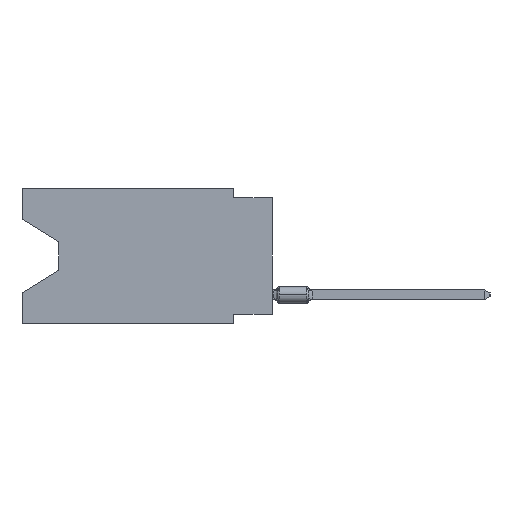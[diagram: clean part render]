
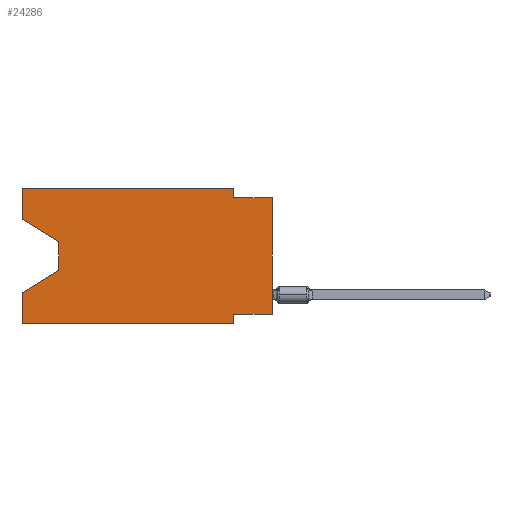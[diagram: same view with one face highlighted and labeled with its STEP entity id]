
A CAD part, left-side view. The second image highlights one B-rep face of the part: STEP entity #24286.
In plain terms, the highlighted planar face has unit normal (-1, 0, 0).
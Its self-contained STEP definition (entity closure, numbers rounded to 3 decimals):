
#262 = VECTOR ( 'NONE', #4071, 1000. ) ;
#324 = ORIENTED_EDGE ( 'NONE', *, *, #18573, .F. ) ;
#328 = CARTESIAN_POINT ( 'NONE',  ( 0., 16.383, -2.038 ) ) ;
#471 = LINE ( 'NONE', #13363, #9251 ) ;
#623 = PLANE ( 'NONE',  #5775 ) ;
#1856 = LINE ( 'NONE', #10464, #262 ) ;
#2342 = EDGE_CURVE ( 'NONE', #5266, #21382, #18797, .T. ) ;
#2840 = CARTESIAN_POINT ( 'NONE',  ( 0., 2.54, 0. ) ) ;
#3054 = LINE ( 'NONE', #19985, #20919 ) ;
#3543 = DIRECTION ( 'NONE',  ( 0., 0., -1. ) ) ;
#4071 = DIRECTION ( 'NONE',  ( 0., 0., 1. ) ) ;
#4153 = CARTESIAN_POINT ( 'NONE',  ( 0., 13.97, -5.385 ) ) ;
#4239 = DIRECTION ( 'NONE',  ( 0., 1., 0. ) ) ;
#4320 = CARTESIAN_POINT ( 'NONE',  ( 0., 0., -0.635 ) ) ;
#4401 = VERTEX_POINT ( 'NONE', #4153 ) ;
#4506 = CARTESIAN_POINT ( 'NONE',  ( 0., 2.54, -8.255 ) ) ;
#4637 = FACE_OUTER_BOUND ( 'NONE', #16215, .T. ) ;
#5173 = EDGE_CURVE ( 'NONE', #19352, #20812, #471, .T. ) ;
#5266 = VERTEX_POINT ( 'NONE', #328 ) ;
#5278 = VECTOR ( 'NONE', #3543, 1000. ) ;
#5775 = AXIS2_PLACEMENT_3D ( 'NONE', #13106, #11027, #21830 ) ;
#6265 = CARTESIAN_POINT ( 'NONE',  ( 0., 16.383, 0. ) ) ;
#6317 = DIRECTION ( 'NONE',  ( 0., -0.855, -0.519 ) ) ;
#6506 = VECTOR ( 'NONE', #14333, 1000. ) ;
#6592 = ORIENTED_EDGE ( 'NONE', *, *, #15731, .T. ) ;
#7139 = VECTOR ( 'NONE', #4239, 1000. ) ;
#7434 = LINE ( 'NONE', #18246, #5278 ) ;
#7458 = EDGE_CURVE ( 'NONE', #15895, #26619, #1856, .T. ) ;
#7667 = CARTESIAN_POINT ( 'NONE',  ( 0., 16.383, 0. ) ) ;
#7800 = LINE ( 'NONE', #11977, #6506 ) ;
#7867 = CARTESIAN_POINT ( 'NONE',  ( 0., 16.383, -8.89 ) ) ;
#8213 = ORIENTED_EDGE ( 'NONE', *, *, #8939, .F. ) ;
#8368 = LINE ( 'NONE', #10178, #14733 ) ;
#8939 = EDGE_CURVE ( 'NONE', #5266, #10581, #8368, .T. ) ;
#8975 = ORIENTED_EDGE ( 'NONE', *, *, #22184, .F. ) ;
#9251 = VECTOR ( 'NONE', #21412, 1000. ) ;
#9270 = VECTOR ( 'NONE', #25116, 1000. ) ;
#9853 = CARTESIAN_POINT ( 'NONE',  ( 0., 2.54, -0.635 ) ) ;
#9855 = CARTESIAN_POINT ( 'NONE',  ( 0., 2.54, -8.89 ) ) ;
#10178 = CARTESIAN_POINT ( 'NONE',  ( 0., 16.383, 0. ) ) ;
#10286 = EDGE_CURVE ( 'NONE', #10581, #26738, #18322, .T. ) ;
#10464 = CARTESIAN_POINT ( 'NONE',  ( 0., 0., 0. ) ) ;
#10512 = EDGE_CURVE ( 'NONE', #19696, #26619, #23321, .T. ) ;
#10581 = VERTEX_POINT ( 'NONE', #7667 ) ;
#10823 = VECTOR ( 'NONE', #12796, 1000. ) ;
#11027 = DIRECTION ( 'NONE',  ( 1., 0., 0. ) ) ;
#11950 = ORIENTED_EDGE ( 'NONE', *, *, #10286, .F. ) ;
#11977 = CARTESIAN_POINT ( 'NONE',  ( 0., 13.97, -5.385 ) ) ;
#12538 = DIRECTION ( 'NONE',  ( 0., 0., 1. ) ) ;
#12659 = LINE ( 'NONE', #6265, #9270 ) ;
#12776 = ORIENTED_EDGE ( 'NONE', *, *, #2342, .T. ) ;
#12796 = DIRECTION ( 'NONE',  ( 0., -1., 0. ) ) ;
#13106 = CARTESIAN_POINT ( 'NONE',  ( 0., 16.383, 0. ) ) ;
#13363 = CARTESIAN_POINT ( 'NONE',  ( 0., 16.383, -8.89 ) ) ;
#13785 = LINE ( 'NONE', #18331, #18627 ) ;
#14333 = DIRECTION ( 'NONE',  ( 0., 0.855, -0.519 ) ) ;
#14733 = VECTOR ( 'NONE', #12538, 1000. ) ;
#15122 = ORIENTED_EDGE ( 'NONE', *, *, #20645, .F. ) ;
#15731 = EDGE_CURVE ( 'NONE', #4401, #20857, #7800, .T. ) ;
#15895 = VERTEX_POINT ( 'NONE', #27357 ) ;
#16215 = EDGE_LOOP ( 'NONE', ( #12776, #17631, #6592, #8975, #17224, #324, #15122, #19209, #16489, #25407, #11950, #8213 ) ) ;
#16489 = ORIENTED_EDGE ( 'NONE', *, *, #10512, .F. ) ;
#17175 = CARTESIAN_POINT ( 'NONE',  ( 0., 13.97, -3.505 ) ) ;
#17224 = ORIENTED_EDGE ( 'NONE', *, *, #5173, .T. ) ;
#17631 = ORIENTED_EDGE ( 'NONE', *, *, #21135, .T. ) ;
#18037 = VECTOR ( 'NONE', #6317, 1000. ) ;
#18246 = CARTESIAN_POINT ( 'NONE',  ( 0., 2.54, -8.89 ) ) ;
#18322 = LINE ( 'NONE', #22482, #24961 ) ;
#18331 = CARTESIAN_POINT ( 'NONE',  ( 0., 2.54, 0. ) ) ;
#18444 = CARTESIAN_POINT ( 'NONE',  ( 0., 16.383, -6.852 ) ) ;
#18573 = EDGE_CURVE ( 'NONE', #26649, #20812, #7434, .T. ) ;
#18627 = VECTOR ( 'NONE', #20428, 1000. ) ;
#18797 = LINE ( 'NONE', #21169, #18037 ) ;
#19209 = ORIENTED_EDGE ( 'NONE', *, *, #7458, .T. ) ;
#19352 = VERTEX_POINT ( 'NONE', #7867 ) ;
#19696 = VERTEX_POINT ( 'NONE', #9853 ) ;
#19985 = CARTESIAN_POINT ( 'NONE',  ( 0., 13.97, -3.505 ) ) ;
#20428 = DIRECTION ( 'NONE',  ( 0., 0., -1. ) ) ;
#20645 = EDGE_CURVE ( 'NONE', #15895, #26649, #22805, .T. ) ;
#20812 = VERTEX_POINT ( 'NONE', #9855 ) ;
#20857 = VERTEX_POINT ( 'NONE', #18444 ) ;
#20919 = VECTOR ( 'NONE', #21778, 1000. ) ;
#21135 = EDGE_CURVE ( 'NONE', #21382, #4401, #3054, .T. ) ;
#21169 = CARTESIAN_POINT ( 'NONE',  ( 0., 16.383, -2.038 ) ) ;
#21382 = VERTEX_POINT ( 'NONE', #17175 ) ;
#21412 = DIRECTION ( 'NONE',  ( 0., -1., 0. ) ) ;
#21778 = DIRECTION ( 'NONE',  ( 0., 0., -1. ) ) ;
#21830 = DIRECTION ( 'NONE',  ( 0., 0., -1. ) ) ;
#22184 = EDGE_CURVE ( 'NONE', #19352, #20857, #12659, .T. ) ;
#22482 = CARTESIAN_POINT ( 'NONE',  ( 0., 16.383, 0. ) ) ;
#22805 = LINE ( 'NONE', #25315, #7139 ) ;
#23231 = CARTESIAN_POINT ( 'NONE',  ( 0., 0., -0.635 ) ) ;
#23321 = LINE ( 'NONE', #4320, #10823 ) ;
#24286 = ADVANCED_FACE ( 'NONE', ( #4637 ), #623, .F. ) ;
#24303 = DIRECTION ( 'NONE',  ( 0., -1., 0. ) ) ;
#24423 = EDGE_CURVE ( 'NONE', #26738, #19696, #13785, .T. ) ;
#24961 = VECTOR ( 'NONE', #24303, 1000. ) ;
#25116 = DIRECTION ( 'NONE',  ( 0., 0., 1. ) ) ;
#25315 = CARTESIAN_POINT ( 'NONE',  ( 0., 0., -8.255 ) ) ;
#25407 = ORIENTED_EDGE ( 'NONE', *, *, #24423, .F. ) ;
#26619 = VERTEX_POINT ( 'NONE', #23231 ) ;
#26649 = VERTEX_POINT ( 'NONE', #4506 ) ;
#26738 = VERTEX_POINT ( 'NONE', #2840 ) ;
#27357 = CARTESIAN_POINT ( 'NONE',  ( 0., 0., -8.255 ) ) ;
